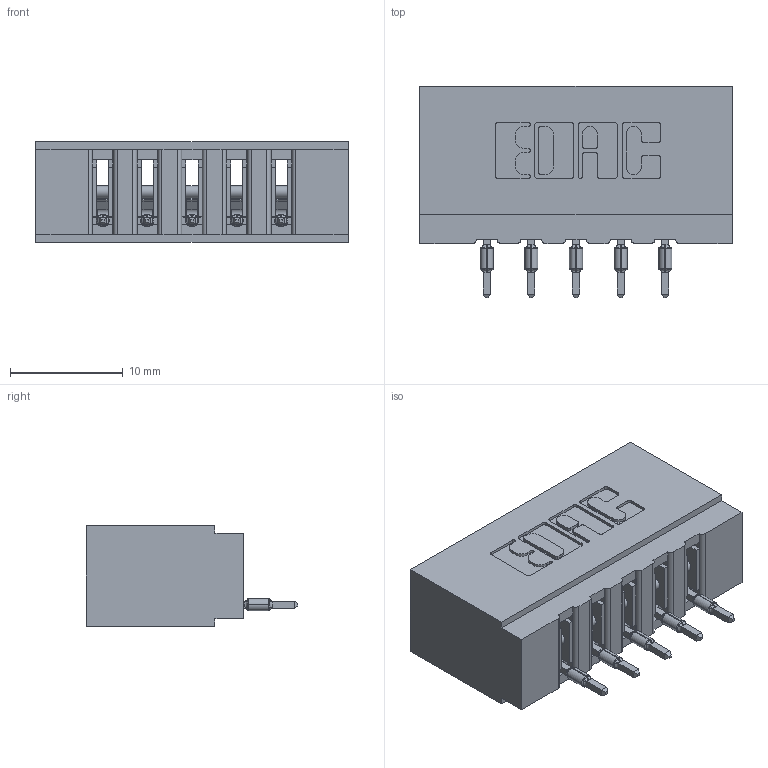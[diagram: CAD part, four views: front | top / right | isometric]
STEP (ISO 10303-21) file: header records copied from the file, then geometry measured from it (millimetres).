
FILE_DESCRIPTION (( 'STEP AP203' ), '1' );
FILE_NAME ('717-005-560-106.STEP', '2020-03-13T17:36:08', ( '' ), ( '' ), 'SwSTEP 2.0', 'SolidWorks 2016', '' );
FILE_SCHEMA (( 'CONFIG_CONTROL_DESIGN' ));
Length unit declared in the file: inch
Products named in the file (3): 717-005-560-106; 745-292-001_560; 717 Part_Insulator Option - 06
Assembly tree (6 placements, depth 2):
  717-005-560-106
    717 Part_Insulator Option - 06
    745-292-001_560  x5
Bounding box: 27.69 x 18.78 x 8.89 mm (x, y, z)
Volume: 2521.5 mm3; surface area: 3220.4 mm2
Topology: 6 solids, 6 shells, 704 faces, 1951 edges, 1246 vertices
Faces by surface type: plane 419, cylinder 155, bspline 100, torus 30
Entity records: 13734 total; most frequent: CARTESIAN_POINT 2920, ORIENTED_EDGE 2286, DIRECTION 2025, EDGE_CURVE 1143, VECTOR 923, LINE 923, VERTEX_POINT 734, AXIS2_PLACEMENT_3D 551
